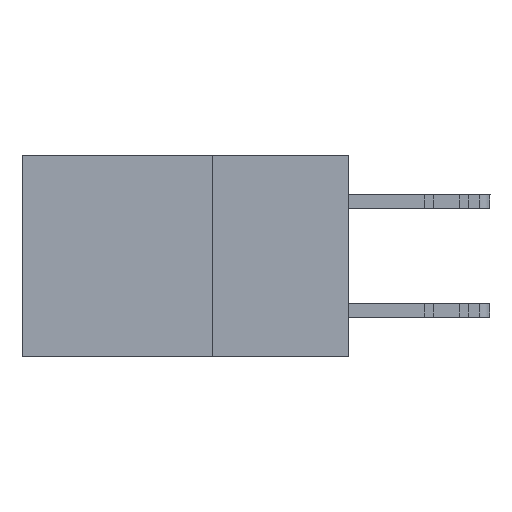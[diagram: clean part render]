
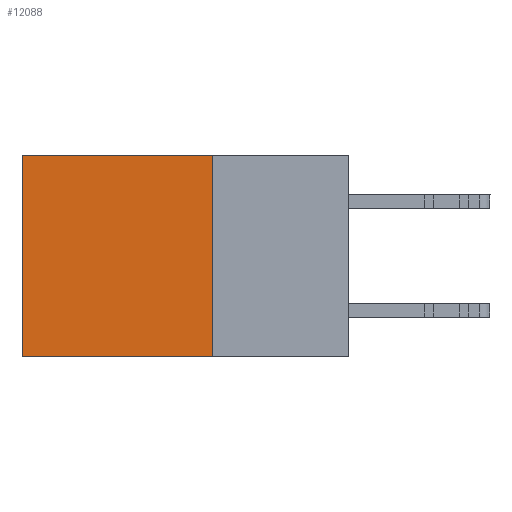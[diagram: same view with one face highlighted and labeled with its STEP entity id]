
A CAD part, left-side view. The second image highlights one B-rep face of the part: STEP entity #12088.
In plain terms, the highlighted planar face has unit normal (-1, 0, 0).
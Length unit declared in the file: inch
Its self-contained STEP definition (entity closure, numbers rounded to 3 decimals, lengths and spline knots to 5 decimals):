
#1144 = CARTESIAN_POINT ( 'NONE',  ( 0.298, 0.25, 0. ) ) ;
#2219 = CARTESIAN_POINT ( 'NONE',  ( 0.298, 0.25, 0. ) ) ;
#3182 = DIRECTION ( 'NONE',  ( 0., 1., 0. ) ) ;
#3828 = LINE ( 'NONE', #18061, #22628 ) ;
#3886 = CARTESIAN_POINT ( 'NONE',  ( 0.298, 0.6, 0. ) ) ;
#6470 = ORIENTED_EDGE ( 'NONE', *, *, #8011, .F. ) ;
#6722 = CARTESIAN_POINT ( 'NONE',  ( 0.298, 0.6, -0.37 ) ) ;
#7055 = VERTEX_POINT ( 'NONE', #2219 ) ;
#7277 = CARTESIAN_POINT ( 'NONE',  ( 0.298, 0.25, -0.37 ) ) ;
#8011 = EDGE_CURVE ( 'NONE', #21078, #16726, #13529, .T. ) ;
#8406 = LINE ( 'NONE', #1144, #10595 ) ;
#8546 = ORIENTED_EDGE ( 'NONE', *, *, #25690, .T. ) ;
#9086 = VECTOR ( 'NONE', #15493, 39.37008 ) ;
#10307 = AXIS2_PLACEMENT_3D ( 'NONE', #15777, #15600, #10895 ) ;
#10595 = VECTOR ( 'NONE', #21032, 39.37008 ) ;
#10895 = DIRECTION ( 'NONE',  ( 0., 0., -1. ) ) ;
#10979 = EDGE_CURVE ( 'NONE', #27523, #16726, #3828, .T. ) ;
#12088 = ADVANCED_FACE ( 'NONE', ( #20120 ), #12848, .F. ) ;
#12848 = PLANE ( 'NONE',  #10307 ) ;
#13004 = DIRECTION ( 'NONE',  ( 0., 0., -1. ) ) ;
#13529 = LINE ( 'NONE', #25301, #31459 ) ;
#15493 = DIRECTION ( 'NONE',  ( 0., 0., -1. ) ) ;
#15600 = DIRECTION ( 'NONE',  ( 1., 0., 0. ) ) ;
#15777 = CARTESIAN_POINT ( 'NONE',  ( 0.298, 0.25, 0. ) ) ;
#15988 = ORIENTED_EDGE ( 'NONE', *, *, #17415, .F. ) ;
#16726 = VERTEX_POINT ( 'NONE', #6722 ) ;
#17355 = CARTESIAN_POINT ( 'NONE',  ( 0.298, 0.25, 0. ) ) ;
#17415 = EDGE_CURVE ( 'NONE', #7055, #21078, #25352, .T. ) ;
#18061 = CARTESIAN_POINT ( 'NONE',  ( 0.298, 0.6, 0. ) ) ;
#20083 = ORIENTED_EDGE ( 'NONE', *, *, #10979, .T. ) ;
#20120 = FACE_OUTER_BOUND ( 'NONE', #27945, .T. ) ;
#21032 = DIRECTION ( 'NONE',  ( 0., 1., 0. ) ) ;
#21078 = VERTEX_POINT ( 'NONE', #7277 ) ;
#22628 = VECTOR ( 'NONE', #13004, 39.37008 ) ;
#25301 = CARTESIAN_POINT ( 'NONE',  ( 0.298, 0.25, -0.37 ) ) ;
#25352 = LINE ( 'NONE', #17355, #9086 ) ;
#25690 = EDGE_CURVE ( 'NONE', #7055, #27523, #8406, .T. ) ;
#27523 = VERTEX_POINT ( 'NONE', #3886 ) ;
#27945 = EDGE_LOOP ( 'NONE', ( #20083, #6470, #15988, #8546 ) ) ;
#31459 = VECTOR ( 'NONE', #3182, 39.37008 ) ;
